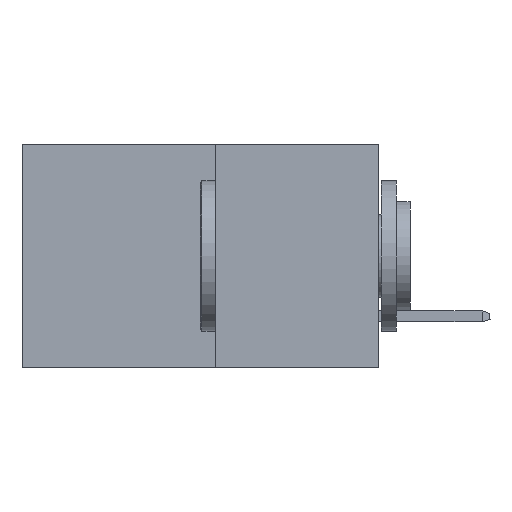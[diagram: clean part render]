
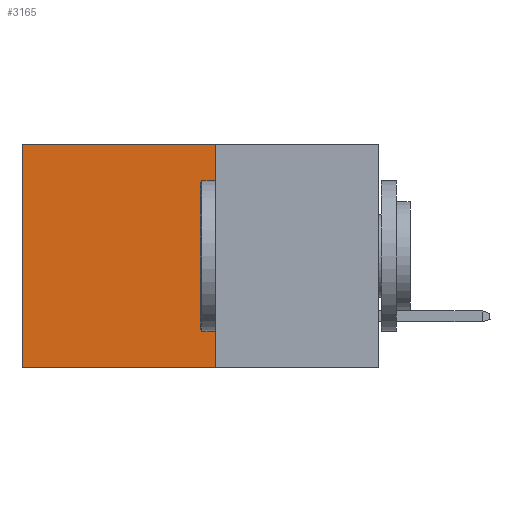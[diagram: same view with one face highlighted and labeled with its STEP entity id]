
A CAD part, left-side view. The second image highlights one B-rep face of the part: STEP entity #3165.
In plain terms, the highlighted planar face has unit normal (-1, 0, 0).
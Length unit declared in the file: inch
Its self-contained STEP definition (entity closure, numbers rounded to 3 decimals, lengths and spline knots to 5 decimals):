
#822 = CARTESIAN_POINT ( 'NONE',  ( 0.277, 0.27, -0.37 ) ) ;
#1770 = CARTESIAN_POINT ( 'NONE',  ( 0.277, 0.59, -0.37 ) ) ;
#2556 = FACE_OUTER_BOUND ( 'NONE', #2570, .T. ) ;
#2570 = EDGE_LOOP ( 'NONE', ( #10419, #13616, #11183, #11547 ) ) ;
#3165 = ADVANCED_FACE ( 'NONE', ( #2556 ), #10805, .F. ) ;
#3179 = EDGE_CURVE ( 'NONE', #10048, #7379, #5094, .T. ) ;
#3523 = VERTEX_POINT ( 'NONE', #8193 ) ;
#3598 = VECTOR ( 'NONE', #4077, 39.37008 ) ;
#4077 = DIRECTION ( 'NONE',  ( 0., 0., -1. ) ) ;
#4087 = CARTESIAN_POINT ( 'NONE',  ( 0.277, 0.59, -0.37 ) ) ;
#4093 = EDGE_CURVE ( 'NONE', #5452, #3523, #12854, .T. ) ;
#4136 = CARTESIAN_POINT ( 'NONE',  ( 0.277, 0.27, -0.37 ) ) ;
#4387 = LINE ( 'NONE', #4136, #3598 ) ;
#4593 = EDGE_CURVE ( 'NONE', #5452, #10048, #4387, .T. ) ;
#5094 = LINE ( 'NONE', #10767, #8094 ) ;
#5213 = LINE ( 'NONE', #1770, #11456 ) ;
#5452 = VERTEX_POINT ( 'NONE', #7903 ) ;
#6687 = CARTESIAN_POINT ( 'NONE',  ( 0.277, 0.27, 0. ) ) ;
#6931 = DIRECTION ( 'NONE',  ( 0., 0., -1. ) ) ;
#7379 = VERTEX_POINT ( 'NONE', #4087 ) ;
#7903 = CARTESIAN_POINT ( 'NONE',  ( 0.277, 0.27, 0. ) ) ;
#8094 = VECTOR ( 'NONE', #9750, 39.37008 ) ;
#8193 = CARTESIAN_POINT ( 'NONE',  ( 0.277, 0.59, 0. ) ) ;
#8603 = AXIS2_PLACEMENT_3D ( 'NONE', #9642, #10941, #9762 ) ;
#9618 = VECTOR ( 'NONE', #11797, 39.37008 ) ;
#9642 = CARTESIAN_POINT ( 'NONE',  ( 0.277, 0.27, -0.37 ) ) ;
#9750 = DIRECTION ( 'NONE',  ( 0., 1., 0. ) ) ;
#9762 = DIRECTION ( 'NONE',  ( 0., 0., -1. ) ) ;
#10048 = VERTEX_POINT ( 'NONE', #822 ) ;
#10419 = ORIENTED_EDGE ( 'NONE', *, *, #12231, .T. ) ;
#10767 = CARTESIAN_POINT ( 'NONE',  ( 0.277, 0.27, -0.37 ) ) ;
#10805 = PLANE ( 'NONE',  #8603 ) ;
#10941 = DIRECTION ( 'NONE',  ( 1., 0., 0. ) ) ;
#11183 = ORIENTED_EDGE ( 'NONE', *, *, #4593, .F. ) ;
#11456 = VECTOR ( 'NONE', #6931, 39.37008 ) ;
#11547 = ORIENTED_EDGE ( 'NONE', *, *, #4093, .T. ) ;
#11797 = DIRECTION ( 'NONE',  ( 0., 1., 0. ) ) ;
#12231 = EDGE_CURVE ( 'NONE', #3523, #7379, #5213, .T. ) ;
#12854 = LINE ( 'NONE', #6687, #9618 ) ;
#13616 = ORIENTED_EDGE ( 'NONE', *, *, #3179, .F. ) ;
